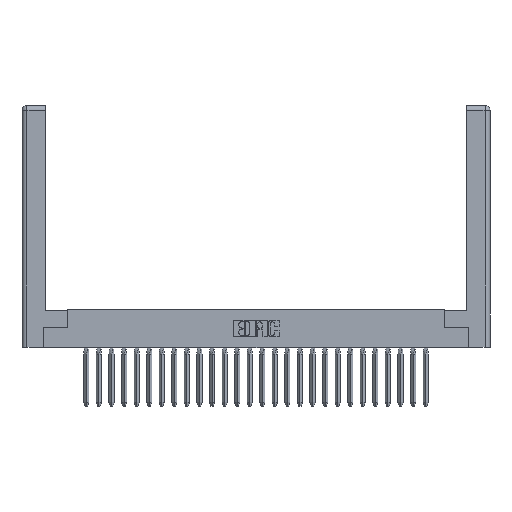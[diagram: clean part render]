
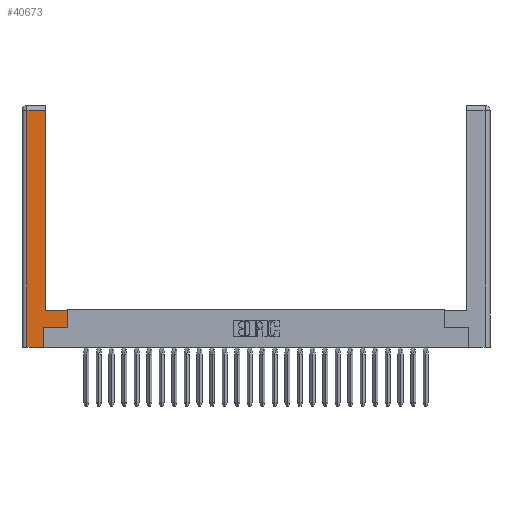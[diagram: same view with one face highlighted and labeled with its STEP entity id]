
A CAD part, top view. The second image highlights one B-rep face of the part: STEP entity #40673.
In plain terms, the highlighted planar face has unit normal (0, 0, 1).
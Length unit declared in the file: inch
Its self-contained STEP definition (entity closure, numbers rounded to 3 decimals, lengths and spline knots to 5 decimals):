
#1136 = CARTESIAN_POINT ( 'NONE',  ( 0.565, 0.45, 0. ) ) ;
#1147 = DIRECTION ( 'NONE',  ( 1., 0., 0. ) ) ;
#2654 = ORIENTED_EDGE ( 'NONE', *, *, #5393, .T. ) ;
#2938 = EDGE_CURVE ( 'NONE', #20155, #14623, #52398, .T. ) ;
#4237 = CARTESIAN_POINT ( 'NONE',  ( 0.295, 0.45, 0. ) ) ;
#4303 = DIRECTION ( 'NONE',  ( 0., 1., 0. ) ) ;
#5111 = LINE ( 'NONE', #1136, #17584 ) ;
#5393 = EDGE_CURVE ( 'NONE', #36104, #20155, #5111, .T. ) ;
#8120 = EDGE_CURVE ( 'NONE', #17769, #36104, #34694, .T. ) ;
#8321 = CARTESIAN_POINT ( 'NONE',  ( 0.565, 0.245, 0. ) ) ;
#9077 = EDGE_CURVE ( 'NONE', #20267, #24170, #53395, .T. ) ;
#10391 = ORIENTED_EDGE ( 'NONE', *, *, #9077, .T. ) ;
#10644 = ORIENTED_EDGE ( 'NONE', *, *, #8120, .T. ) ;
#11414 = VECTOR ( 'NONE', #4303, 39.37008 ) ;
#12576 = DIRECTION ( 'NONE',  ( -1., 0., 0. ) ) ;
#13039 = PLANE ( 'NONE',  #36910 ) ;
#13277 = CARTESIAN_POINT ( 'NONE',  ( 0.0615, 0., 0. ) ) ;
#14623 = VERTEX_POINT ( 'NONE', #4237 ) ;
#14966 = EDGE_CURVE ( 'NONE', #39263, #17769, #29604, .T. ) ;
#15541 = CARTESIAN_POINT ( 'NONE',  ( 0.0615, 0., 0. ) ) ;
#15654 = CARTESIAN_POINT ( 'NONE',  ( 0.295, 0.45, 0. ) ) ;
#16796 = DIRECTION ( 'NONE',  ( -1., 0., 0. ) ) ;
#16884 = DIRECTION ( 'NONE',  ( 0., 0., -1. ) ) ;
#17584 = VECTOR ( 'NONE', #18987, 39.37008 ) ;
#17769 = VERTEX_POINT ( 'NONE', #34758 ) ;
#17876 = DIRECTION ( 'NONE',  ( 0., -1., 0. ) ) ;
#18489 = ORIENTED_EDGE ( 'NONE', *, *, #33715, .T. ) ;
#18987 = DIRECTION ( 'NONE',  ( 0., 1., 0. ) ) ;
#20155 = VERTEX_POINT ( 'NONE', #34652 ) ;
#20267 = VERTEX_POINT ( 'NONE', #27433 ) ;
#21553 = DIRECTION ( 'NONE',  ( -1., 0., 0. ) ) ;
#21975 = FACE_OUTER_BOUND ( 'NONE', #40630, .T. ) ;
#22836 = VECTOR ( 'NONE', #23731, 39.37008 ) ;
#23731 = DIRECTION ( 'NONE',  ( 1., 0., 0. ) ) ;
#23854 = ORIENTED_EDGE ( 'NONE', *, *, #28850, .T. ) ;
#24170 = VERTEX_POINT ( 'NONE', #41504 ) ;
#24415 = LINE ( 'NONE', #13277, #34200 ) ;
#24493 = LINE ( 'NONE', #41564, #49633 ) ;
#27433 = CARTESIAN_POINT ( 'NONE',  ( 0.295, 2.94, 0. ) ) ;
#28405 = VERTEX_POINT ( 'NONE', #15541 ) ;
#28653 = VECTOR ( 'NONE', #16796, 39.37008 ) ;
#28850 = EDGE_CURVE ( 'NONE', #28405, #39263, #24493, .T. ) ;
#29604 = LINE ( 'NONE', #33557, #44934 ) ;
#33024 = ORIENTED_EDGE ( 'NONE', *, *, #41888, .T. ) ;
#33557 = CARTESIAN_POINT ( 'NONE',  ( 0.265, 0.245, 0. ) ) ;
#33715 = EDGE_CURVE ( 'NONE', #24170, #28405, #24415, .T. ) ;
#34200 = VECTOR ( 'NONE', #17876, 39.37008 ) ;
#34373 = LINE ( 'NONE', #57676, #11414 ) ;
#34652 = CARTESIAN_POINT ( 'NONE',  ( 0.565, 0.45, 0. ) ) ;
#34694 = LINE ( 'NONE', #55147, #22836 ) ;
#34758 = CARTESIAN_POINT ( 'NONE',  ( 0.265, 0.245, 0. ) ) ;
#34797 = CARTESIAN_POINT ( 'NONE',  ( 0.265, 0., 0. ) ) ;
#36104 = VERTEX_POINT ( 'NONE', #8321 ) ;
#36910 = AXIS2_PLACEMENT_3D ( 'NONE', #44135, #16884, #21553 ) ;
#39263 = VERTEX_POINT ( 'NONE', #34797 ) ;
#40630 = EDGE_LOOP ( 'NONE', ( #33024, #10391, #18489, #23854, #51429, #10644, #2654, #41720 ) ) ;
#40673 = ADVANCED_FACE ( 'NONE', ( #21975 ), #13039, .F. ) ;
#41481 = VECTOR ( 'NONE', #12576, 39.37008 ) ;
#41504 = CARTESIAN_POINT ( 'NONE',  ( 0.0615, 2.94, 0. ) ) ;
#41564 = CARTESIAN_POINT ( 'NONE',  ( 0.265, 0., 0. ) ) ;
#41720 = ORIENTED_EDGE ( 'NONE', *, *, #2938, .T. ) ;
#41888 = EDGE_CURVE ( 'NONE', #14623, #20267, #34373, .T. ) ;
#44135 = CARTESIAN_POINT ( 'NONE',  ( 0., 0., 0. ) ) ;
#44934 = VECTOR ( 'NONE', #48031, 39.37008 ) ;
#48031 = DIRECTION ( 'NONE',  ( 0., 1., 0. ) ) ;
#48197 = CARTESIAN_POINT ( 'NONE',  ( 0.0615, 2.94, 0. ) ) ;
#49633 = VECTOR ( 'NONE', #1147, 39.37008 ) ;
#51429 = ORIENTED_EDGE ( 'NONE', *, *, #14966, .T. ) ;
#52398 = LINE ( 'NONE', #15654, #28653 ) ;
#53395 = LINE ( 'NONE', #48197, #41481 ) ;
#55147 = CARTESIAN_POINT ( 'NONE',  ( 0.565, 0.245, 0. ) ) ;
#57676 = CARTESIAN_POINT ( 'NONE',  ( 0.295, 3., 0. ) ) ;
